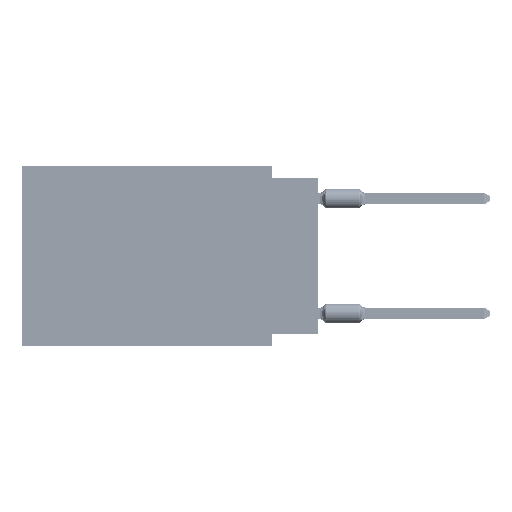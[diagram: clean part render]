
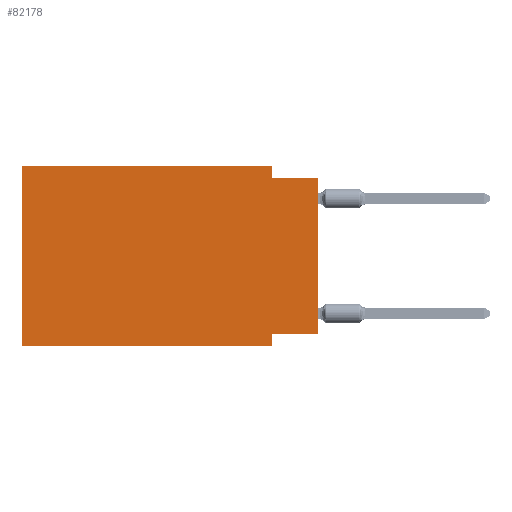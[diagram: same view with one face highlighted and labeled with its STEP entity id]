
A CAD part, left-side view. The second image highlights one B-rep face of the part: STEP entity #82178.
In plain terms, the highlighted planar face has unit normal (-1, 0, 0).
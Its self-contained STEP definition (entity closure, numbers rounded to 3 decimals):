
#321 = EDGE_LOOP ( 'NONE', ( #63567, #60009, #50028, #38148, #40440, #20661, #23169, #52020 ) ) ;
#1835 = LINE ( 'NONE', #19205, #46980 ) ;
#3054 = LINE ( 'NONE', #10130, #64241 ) ;
#8343 = LINE ( 'NONE', #33487, #47693 ) ;
#8387 = VECTOR ( 'NONE', #80876, 1000. ) ;
#9764 = DIRECTION ( 'NONE',  ( 0., -1., 0. ) ) ;
#9997 = DIRECTION ( 'NONE',  ( 0., 0., -1. ) ) ;
#10130 = CARTESIAN_POINT ( 'NONE',  ( 0., 16.383, 0. ) ) ;
#12488 = CARTESIAN_POINT ( 'NONE',  ( 0., 2.54, 0. ) ) ;
#14510 = DIRECTION ( 'NONE',  ( 0., 1., 0. ) ) ;
#15029 = EDGE_CURVE ( 'NONE', #40539, #65302, #1835, .T. ) ;
#16231 = VERTEX_POINT ( 'NONE', #44392 ) ;
#16819 = EDGE_CURVE ( 'NONE', #17538, #27726, #72939, .T. ) ;
#17538 = VERTEX_POINT ( 'NONE', #54493 ) ;
#17682 = CARTESIAN_POINT ( 'NONE',  ( 0., 0., -0.635 ) ) ;
#17964 = AXIS2_PLACEMENT_3D ( 'NONE', #35166, #49292, #9997 ) ;
#18002 = EDGE_CURVE ( 'NONE', #16231, #65302, #47327, .T. ) ;
#19205 = CARTESIAN_POINT ( 'NONE',  ( 0., 16.383, -9.906 ) ) ;
#20091 = LINE ( 'NONE', #27552, #70113 ) ;
#20661 = ORIENTED_EDGE ( 'NONE', *, *, #15029, .T. ) ;
#20707 = VECTOR ( 'NONE', #72291, 1000. ) ;
#21396 = DIRECTION ( 'NONE',  ( 0., 0., 1. ) ) ;
#21399 = EDGE_CURVE ( 'NONE', #27726, #68272, #22998, .T. ) ;
#22998 = LINE ( 'NONE', #17682, #79452 ) ;
#23169 = ORIENTED_EDGE ( 'NONE', *, *, #18002, .F. ) ;
#23228 = FACE_OUTER_BOUND ( 'NONE', #321, .T. ) ;
#26576 = EDGE_CURVE ( 'NONE', #32212, #17538, #3054, .T. ) ;
#27552 = CARTESIAN_POINT ( 'NONE',  ( 0., 16.383, 0. ) ) ;
#27726 = VERTEX_POINT ( 'NONE', #52420 ) ;
#32212 = VERTEX_POINT ( 'NONE', #81784 ) ;
#33487 = CARTESIAN_POINT ( 'NONE',  ( 0., 0., -9.271 ) ) ;
#35166 = CARTESIAN_POINT ( 'NONE',  ( 0., 16.383, 0. ) ) ;
#38148 = ORIENTED_EDGE ( 'NONE', *, *, #26576, .F. ) ;
#38314 = EDGE_CURVE ( 'NONE', #79207, #16231, #8343, .T. ) ;
#39389 = DIRECTION ( 'NONE',  ( 0., 0., -1. ) ) ;
#40440 = ORIENTED_EDGE ( 'NONE', *, *, #83785, .F. ) ;
#40539 = VERTEX_POINT ( 'NONE', #73795 ) ;
#44141 = VECTOR ( 'NONE', #39389, 1000. ) ;
#44392 = CARTESIAN_POINT ( 'NONE',  ( 0., 2.54, -9.271 ) ) ;
#46980 = VECTOR ( 'NONE', #47749, 1000. ) ;
#47327 = LINE ( 'NONE', #60589, #8387 ) ;
#47693 = VECTOR ( 'NONE', #14510, 1000. ) ;
#47749 = DIRECTION ( 'NONE',  ( 0., -1., 0. ) ) ;
#49292 = DIRECTION ( 'NONE',  ( 1., 0., 0. ) ) ;
#50028 = ORIENTED_EDGE ( 'NONE', *, *, #16819, .F. ) ;
#52020 = ORIENTED_EDGE ( 'NONE', *, *, #38314, .F. ) ;
#52420 = CARTESIAN_POINT ( 'NONE',  ( 0., 2.54, -0.635 ) ) ;
#54493 = CARTESIAN_POINT ( 'NONE',  ( 0., 2.54, 0. ) ) ;
#57208 = PLANE ( 'NONE',  #17964 ) ;
#60009 = ORIENTED_EDGE ( 'NONE', *, *, #21399, .F. ) ;
#60589 = CARTESIAN_POINT ( 'NONE',  ( 0., 2.54, -9.906 ) ) ;
#60768 = CARTESIAN_POINT ( 'NONE',  ( 0., 0., -0.635 ) ) ;
#63567 = ORIENTED_EDGE ( 'NONE', *, *, #83233, .T. ) ;
#64241 = VECTOR ( 'NONE', #83823, 1000. ) ;
#65302 = VERTEX_POINT ( 'NONE', #65594 ) ;
#65594 = CARTESIAN_POINT ( 'NONE',  ( 0., 2.54, -9.906 ) ) ;
#68272 = VERTEX_POINT ( 'NONE', #60768 ) ;
#70113 = VECTOR ( 'NONE', #21396, 1000. ) ;
#72291 = DIRECTION ( 'NONE',  ( 0., 0., 1. ) ) ;
#72725 = CARTESIAN_POINT ( 'NONE',  ( 0., 0., 0. ) ) ;
#72939 = LINE ( 'NONE', #12488, #44141 ) ;
#73795 = CARTESIAN_POINT ( 'NONE',  ( 0., 16.383, -9.906 ) ) ;
#76562 = CARTESIAN_POINT ( 'NONE',  ( 0., 0., -9.271 ) ) ;
#79207 = VERTEX_POINT ( 'NONE', #76562 ) ;
#79452 = VECTOR ( 'NONE', #9764, 1000. ) ;
#80217 = LINE ( 'NONE', #72725, #20707 ) ;
#80876 = DIRECTION ( 'NONE',  ( 0., 0., -1. ) ) ;
#81784 = CARTESIAN_POINT ( 'NONE',  ( 0., 16.383, 0. ) ) ;
#82178 = ADVANCED_FACE ( 'NONE', ( #23228 ), #57208, .F. ) ;
#83233 = EDGE_CURVE ( 'NONE', #79207, #68272, #80217, .T. ) ;
#83785 = EDGE_CURVE ( 'NONE', #40539, #32212, #20091, .T. ) ;
#83823 = DIRECTION ( 'NONE',  ( 0., -1., 0. ) ) ;
